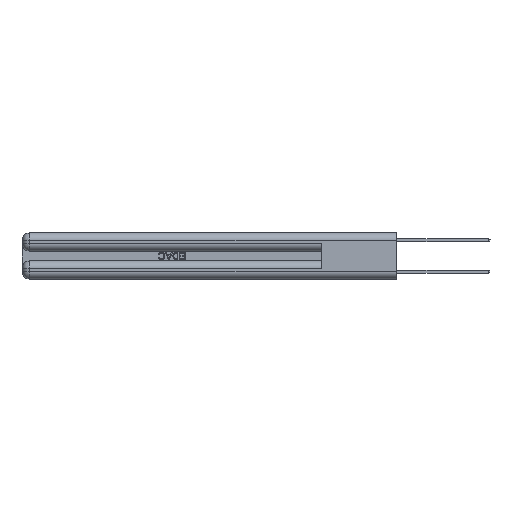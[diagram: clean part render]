
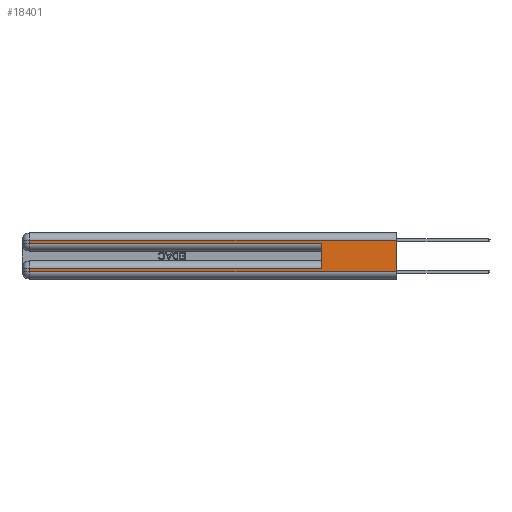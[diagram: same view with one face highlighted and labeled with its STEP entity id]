
A CAD part, left-side view. The second image highlights one B-rep face of the part: STEP entity #18401.
In plain terms, the highlighted planar face has unit normal (-1, 0, 0).
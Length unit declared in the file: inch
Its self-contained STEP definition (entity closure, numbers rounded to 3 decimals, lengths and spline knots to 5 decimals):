
#984 = CARTESIAN_POINT ( 'NONE',  ( 0., 2.94, 0.37 ) ) ;
#1619 = CARTESIAN_POINT ( 'NONE',  ( 0., 0., 0.37 ) ) ;
#2252 = VERTEX_POINT ( 'NONE', #11601 ) ;
#3012 = ORIENTED_EDGE ( 'NONE', *, *, #12389, .T. ) ;
#4634 = EDGE_LOOP ( 'NONE', ( #26040, #23545, #3012, #32368, #22366, #10102, #14052, #8999 ) ) ;
#6353 = CARTESIAN_POINT ( 'NONE',  ( 0., 0.6, 0.285 ) ) ;
#6805 = EDGE_CURVE ( 'NONE', #2252, #23562, #7423, .T. ) ;
#7224 = EDGE_CURVE ( 'NONE', #7571, #10299, #12303, .T. ) ;
#7423 = LINE ( 'NONE', #8035, #27230 ) ;
#7571 = VERTEX_POINT ( 'NONE', #28884 ) ;
#7639 = DIRECTION ( 'NONE',  ( 0., 0., -1. ) ) ;
#7765 = LINE ( 'NONE', #34059, #16827 ) ;
#8035 = CARTESIAN_POINT ( 'NONE',  ( 0., 0., 0.31 ) ) ;
#8999 = ORIENTED_EDGE ( 'NONE', *, *, #31344, .T. ) ;
#9354 = PLANE ( 'NONE',  #10022 ) ;
#10022 = AXIS2_PLACEMENT_3D ( 'NONE', #25308, #11991, #7639 ) ;
#10102 = ORIENTED_EDGE ( 'NONE', *, *, #7224, .T. ) ;
#10299 = VERTEX_POINT ( 'NONE', #30864 ) ;
#10389 = DIRECTION ( 'NONE',  ( 0., -1., 0. ) ) ;
#10665 = VERTEX_POINT ( 'NONE', #6353 ) ;
#10948 = EDGE_CURVE ( 'NONE', #7571, #10665, #31930, .T. ) ;
#11454 = VECTOR ( 'NONE', #20380, 39.37008 ) ;
#11601 = CARTESIAN_POINT ( 'NONE',  ( 0., 0., 0.31 ) ) ;
#11991 = DIRECTION ( 'NONE',  ( 1., 0., 0. ) ) ;
#12303 = LINE ( 'NONE', #25442, #11454 ) ;
#12389 = EDGE_CURVE ( 'NONE', #23562, #13122, #18737, .T. ) ;
#12601 = VECTOR ( 'NONE', #14779, 39.37008 ) ;
#13078 = DIRECTION ( 'NONE',  ( 0., 1., 0. ) ) ;
#13094 = VECTOR ( 'NONE', #15243, 39.37008 ) ;
#13122 = VERTEX_POINT ( 'NONE', #29515 ) ;
#13452 = EDGE_CURVE ( 'NONE', #10299, #16975, #23982, .T. ) ;
#14052 = ORIENTED_EDGE ( 'NONE', *, *, #13452, .T. ) ;
#14779 = DIRECTION ( 'NONE',  ( 0., 0., -1. ) ) ;
#15022 = VECTOR ( 'NONE', #22877, 39.37008 ) ;
#15110 = LINE ( 'NONE', #1619, #12601 ) ;
#15243 = DIRECTION ( 'NONE',  ( 0., -1., 0. ) ) ;
#15348 = DIRECTION ( 'NONE',  ( 0., 0., 1. ) ) ;
#16827 = VECTOR ( 'NONE', #10389, 39.37008 ) ;
#16975 = VERTEX_POINT ( 'NONE', #23070 ) ;
#18401 = ADVANCED_FACE ( 'NONE', ( #25813 ), #9354, .F. ) ;
#18737 = LINE ( 'NONE', #20491, #15022 ) ;
#20006 = CARTESIAN_POINT ( 'NONE',  ( 0., 0., 0.06 ) ) ;
#20380 = DIRECTION ( 'NONE',  ( 0., 1., 0. ) ) ;
#20491 = CARTESIAN_POINT ( 'NONE',  ( 0., 2.94, 0.37 ) ) ;
#22366 = ORIENTED_EDGE ( 'NONE', *, *, #10948, .F. ) ;
#22877 = DIRECTION ( 'NONE',  ( 0., 0., -1. ) ) ;
#23070 = CARTESIAN_POINT ( 'NONE',  ( 0., 2.94, 0.06 ) ) ;
#23545 = ORIENTED_EDGE ( 'NONE', *, *, #6805, .T. ) ;
#23562 = VERTEX_POINT ( 'NONE', #26072 ) ;
#23982 = LINE ( 'NONE', #984, #31427 ) ;
#24418 = DIRECTION ( 'NONE',  ( 0., 0., -1. ) ) ;
#25308 = CARTESIAN_POINT ( 'NONE',  ( 0., 0., 0.37 ) ) ;
#25442 = CARTESIAN_POINT ( 'NONE',  ( 0., 0., 0.085 ) ) ;
#25746 = VECTOR ( 'NONE', #15348, 39.37008 ) ;
#25813 = FACE_OUTER_BOUND ( 'NONE', #4634, .T. ) ;
#26040 = ORIENTED_EDGE ( 'NONE', *, *, #26634, .F. ) ;
#26072 = CARTESIAN_POINT ( 'NONE',  ( 0., 2.94, 0.31 ) ) ;
#26634 = EDGE_CURVE ( 'NONE', #2252, #30008, #15110, .T. ) ;
#27230 = VECTOR ( 'NONE', #13078, 39.37008 ) ;
#28884 = CARTESIAN_POINT ( 'NONE',  ( 0., 0.6, 0.085 ) ) ;
#29515 = CARTESIAN_POINT ( 'NONE',  ( 0., 2.94, 0.285 ) ) ;
#30008 = VERTEX_POINT ( 'NONE', #20006 ) ;
#30864 = CARTESIAN_POINT ( 'NONE',  ( 0., 2.94, 0.085 ) ) ;
#31147 = CARTESIAN_POINT ( 'NONE',  ( 0., 0.6, 0.145 ) ) ;
#31344 = EDGE_CURVE ( 'NONE', #16975, #30008, #31712, .T. ) ;
#31427 = VECTOR ( 'NONE', #24418, 39.37008 ) ;
#31508 = EDGE_CURVE ( 'NONE', #13122, #10665, #7765, .T. ) ;
#31712 = LINE ( 'NONE', #33485, #13094 ) ;
#31930 = LINE ( 'NONE', #31147, #25746 ) ;
#32368 = ORIENTED_EDGE ( 'NONE', *, *, #31508, .T. ) ;
#33485 = CARTESIAN_POINT ( 'NONE',  ( 0., 0., 0.06 ) ) ;
#34059 = CARTESIAN_POINT ( 'NONE',  ( 0., 0., 0.285 ) ) ;
